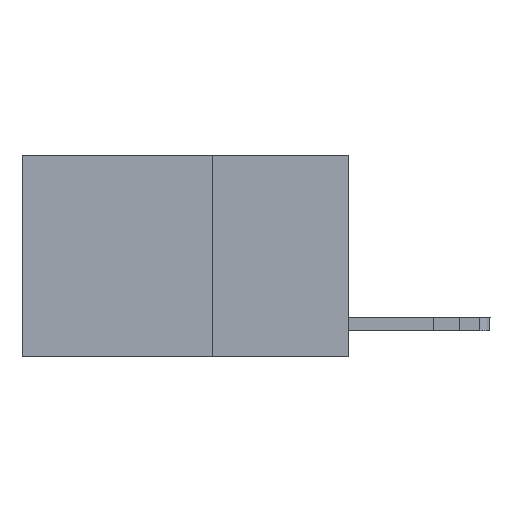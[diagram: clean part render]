
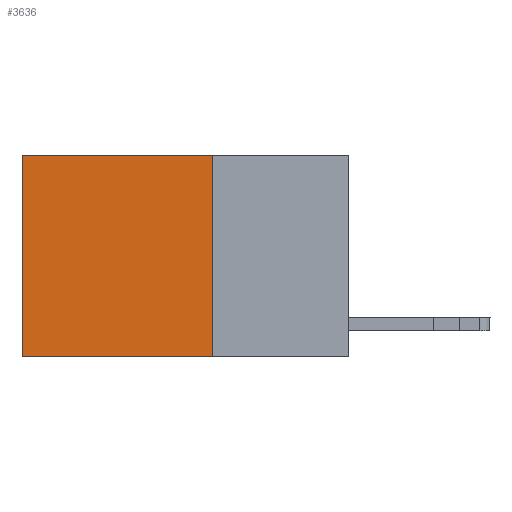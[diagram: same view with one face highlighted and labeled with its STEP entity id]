
A CAD part, left-side view. The second image highlights one B-rep face of the part: STEP entity #3636.
In plain terms, the highlighted planar face has unit normal (-1, 0, 0).
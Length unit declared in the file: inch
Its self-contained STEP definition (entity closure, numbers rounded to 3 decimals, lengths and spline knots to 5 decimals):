
#679 = ORIENTED_EDGE ( 'NONE', *, *, #13717, .T. ) ;
#1023 = EDGE_CURVE ( 'NONE', #3907, #6824, #11968, .T. ) ;
#1187 = ORIENTED_EDGE ( 'NONE', *, *, #1962, .F. ) ;
#1334 = CARTESIAN_POINT ( 'NONE',  ( 0.2625, 0.25, 0. ) ) ;
#1923 = CARTESIAN_POINT ( 'NONE',  ( 0.2625, 0.25, 0. ) ) ;
#1962 = EDGE_CURVE ( 'NONE', #11540, #15399, #15015, .T. ) ;
#3416 = CARTESIAN_POINT ( 'NONE',  ( 0.2625, 0.25, -0.37 ) ) ;
#3636 = ADVANCED_FACE ( 'NONE', ( #6235 ), #16690, .F. ) ;
#3907 = VERTEX_POINT ( 'NONE', #14699 ) ;
#4418 = LINE ( 'NONE', #8386, #15999 ) ;
#5037 = VECTOR ( 'NONE', #9458, 39.37008 ) ;
#6235 = FACE_OUTER_BOUND ( 'NONE', #14229, .T. ) ;
#6637 = DIRECTION ( 'NONE',  ( 1., 0., 0. ) ) ;
#6824 = VERTEX_POINT ( 'NONE', #12516 ) ;
#8162 = ORIENTED_EDGE ( 'NONE', *, *, #9807, .F. ) ;
#8386 = CARTESIAN_POINT ( 'NONE',  ( 0.2625, 0.25, -0.37 ) ) ;
#8783 = VECTOR ( 'NONE', #13080, 39.37008 ) ;
#9458 = DIRECTION ( 'NONE',  ( 0., 0., -1. ) ) ;
#9807 = EDGE_CURVE ( 'NONE', #15399, #6824, #4418, .T. ) ;
#10327 = AXIS2_PLACEMENT_3D ( 'NONE', #15497, #6637, #10781 ) ;
#10419 = LINE ( 'NONE', #1334, #16194 ) ;
#10642 = DIRECTION ( 'NONE',  ( 0., 1., 0. ) ) ;
#10781 = DIRECTION ( 'NONE',  ( 0., 0., -1. ) ) ;
#11540 = VERTEX_POINT ( 'NONE', #14137 ) ;
#11968 = LINE ( 'NONE', #14452, #5037 ) ;
#12199 = DIRECTION ( 'NONE',  ( 0., 1., 0. ) ) ;
#12516 = CARTESIAN_POINT ( 'NONE',  ( 0.2625, 0.6, -0.37 ) ) ;
#13080 = DIRECTION ( 'NONE',  ( 0., 0., -1. ) ) ;
#13717 = EDGE_CURVE ( 'NONE', #11540, #3907, #10419, .T. ) ;
#14137 = CARTESIAN_POINT ( 'NONE',  ( 0.2625, 0.25, 0. ) ) ;
#14229 = EDGE_LOOP ( 'NONE', ( #15606, #8162, #1187, #679 ) ) ;
#14452 = CARTESIAN_POINT ( 'NONE',  ( 0.2625, 0.6, 0. ) ) ;
#14699 = CARTESIAN_POINT ( 'NONE',  ( 0.2625, 0.6, 0. ) ) ;
#15015 = LINE ( 'NONE', #1923, #8783 ) ;
#15399 = VERTEX_POINT ( 'NONE', #3416 ) ;
#15497 = CARTESIAN_POINT ( 'NONE',  ( 0.2625, 0.25, 0. ) ) ;
#15606 = ORIENTED_EDGE ( 'NONE', *, *, #1023, .T. ) ;
#15999 = VECTOR ( 'NONE', #12199, 39.37008 ) ;
#16194 = VECTOR ( 'NONE', #10642, 39.37008 ) ;
#16690 = PLANE ( 'NONE',  #10327 ) ;
